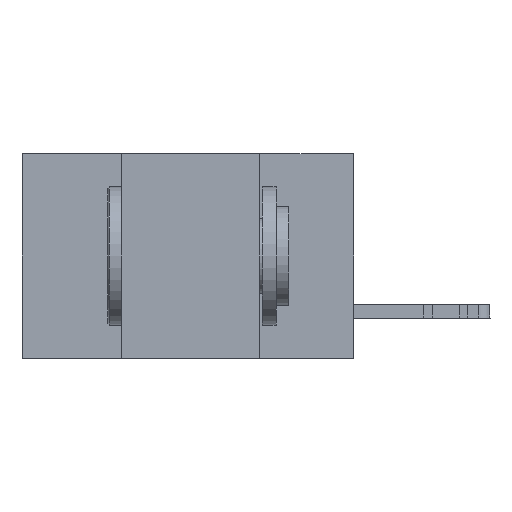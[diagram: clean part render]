
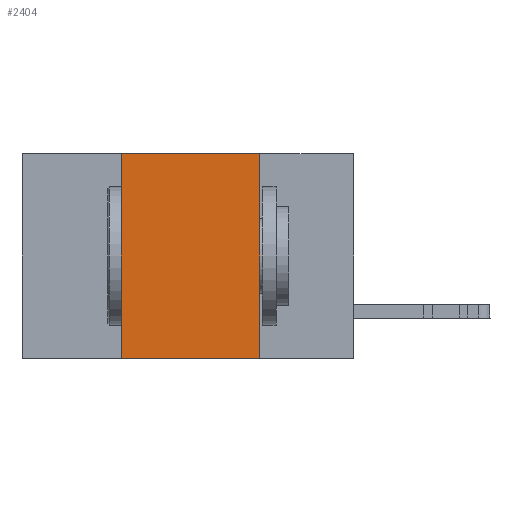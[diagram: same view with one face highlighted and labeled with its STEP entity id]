
A CAD part, left-side view. The second image highlights one B-rep face of the part: STEP entity #2404.
In plain terms, the highlighted planar face has unit normal (-1, 0, 0).
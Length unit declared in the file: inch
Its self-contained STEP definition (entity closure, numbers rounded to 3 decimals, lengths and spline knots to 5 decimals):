
#208 = VERTEX_POINT ( 'NONE', #43795 ) ;
#336 = DIRECTION ( 'NONE',  ( 0., 0., -1. ) ) ;
#703 = LINE ( 'NONE', #25060, #34529 ) ;
#1097 = DIRECTION ( 'NONE',  ( 0., -1., 0. ) ) ;
#1619 = CARTESIAN_POINT ( 'NONE',  ( 0., 0.6, 0. ) ) ;
#2404 = ADVANCED_FACE ( 'NONE', ( #3766 ), #11692, .F. ) ;
#2797 = EDGE_LOOP ( 'NONE', ( #31567, #35943, #22971, #16293 ) ) ;
#3514 = CARTESIAN_POINT ( 'NONE',  ( 0., 0.17, 0. ) ) ;
#3766 = FACE_OUTER_BOUND ( 'NONE', #2797, .T. ) ;
#6408 = VECTOR ( 'NONE', #22403, 39.37008 ) ;
#6416 = CARTESIAN_POINT ( 'NONE',  ( 0., 0.17, 0. ) ) ;
#8053 = CARTESIAN_POINT ( 'NONE',  ( 0., 0.6, 0. ) ) ;
#9152 = EDGE_CURVE ( 'NONE', #22196, #208, #50549, .T. ) ;
#11692 = PLANE ( 'NONE',  #45113 ) ;
#16293 = ORIENTED_EDGE ( 'NONE', *, *, #44719, .T. ) ;
#17852 = CARTESIAN_POINT ( 'NONE',  ( 0., 0.42, 0. ) ) ;
#18037 = LINE ( 'NONE', #49526, #6408 ) ;
#22196 = VERTEX_POINT ( 'NONE', #6416 ) ;
#22403 = DIRECTION ( 'NONE',  ( 0., 0., 1. ) ) ;
#22971 = ORIENTED_EDGE ( 'NONE', *, *, #26417, .F. ) ;
#24730 = DIRECTION ( 'NONE',  ( 0., -1., 0. ) ) ;
#25060 = CARTESIAN_POINT ( 'NONE',  ( 0., 0.6, -0.37 ) ) ;
#26417 = EDGE_CURVE ( 'NONE', #49161, #32649, #18037, .T. ) ;
#29312 = EDGE_CURVE ( 'NONE', #32649, #22196, #36796, .T. ) ;
#31549 = CARTESIAN_POINT ( 'NONE',  ( 0., 0.42, -0.37 ) ) ;
#31567 = ORIENTED_EDGE ( 'NONE', *, *, #9152, .F. ) ;
#32649 = VERTEX_POINT ( 'NONE', #17852 ) ;
#34529 = VECTOR ( 'NONE', #24730, 39.37008 ) ;
#34915 = DIRECTION ( 'NONE',  ( 0., 0., -1. ) ) ;
#35943 = ORIENTED_EDGE ( 'NONE', *, *, #29312, .F. ) ;
#36796 = LINE ( 'NONE', #1619, #45460 ) ;
#39116 = DIRECTION ( 'NONE',  ( 1., 0., 0. ) ) ;
#40085 = VECTOR ( 'NONE', #34915, 39.37008 ) ;
#43795 = CARTESIAN_POINT ( 'NONE',  ( 0., 0.17, -0.37 ) ) ;
#44719 = EDGE_CURVE ( 'NONE', #49161, #208, #703, .T. ) ;
#45113 = AXIS2_PLACEMENT_3D ( 'NONE', #8053, #39116, #336 ) ;
#45460 = VECTOR ( 'NONE', #1097, 39.37008 ) ;
#49161 = VERTEX_POINT ( 'NONE', #31549 ) ;
#49526 = CARTESIAN_POINT ( 'NONE',  ( 0., 0.42, 0. ) ) ;
#50549 = LINE ( 'NONE', #3514, #40085 ) ;
